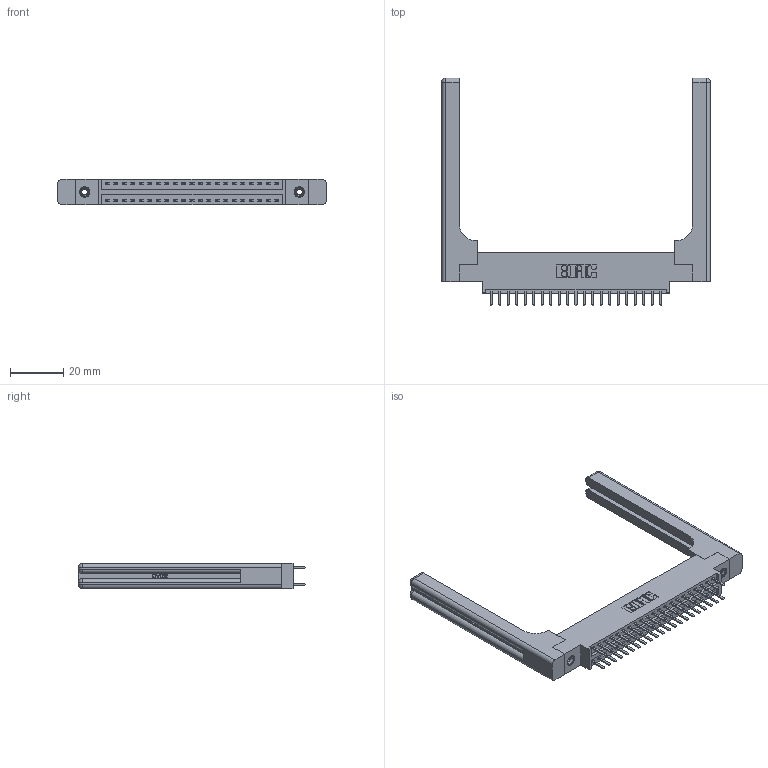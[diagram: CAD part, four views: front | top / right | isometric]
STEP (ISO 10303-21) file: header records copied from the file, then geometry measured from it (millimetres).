
FILE_DESCRIPTION (( 'STEP AP203' ), '1' );
FILE_NAME ('346-042-520-858.STEP', '2022-05-20T03:45:35', ( '' ), ( '' ), 'SwSTEP 2.0', 'SolidWorks 2020', '' );
FILE_SCHEMA (( 'CONFIG_CONTROL_DESIGN' ));
Length unit declared in the file: inch
Products named in the file (5): 346-220-058_345-220-058; 346-042-520-858; 346 Part_0.170 Offset - 0.156 Dia-TH; 345-250-001_345-250-001-102; 345-292-001_345-293-120
Assembly tree (47 placements, depth 2):
  346-042-520-858
    346 Part_0.170 Offset - 0.156 Dia-TH
    345-292-001_345-293-120  x42
    345-250-001_345-250-001-102  x2
    346-220-058_345-220-058  x2
Bounding box: 100.74 x 85.29 x 9.4 mm (x, y, z)
Volume: 16963 mm3; surface area: 17829.1 mm2
Topology: 47 solids, 47 shells, 2748 faces, 7889 edges, 5126 vertices
Faces by surface type: plane 1796, cylinder 892, bspline 36, cone 12, sphere 8, torus 4
Entity records: 22376 total; most frequent: CARTESIAN_POINT 4743, ORIENTED_EDGE 3460, DIRECTION 3150, EDGE_CURVE 1730, LINE 1418, VECTOR 1418, VERTEX_POINT 1142, AXIS2_PLACEMENT_3D 866
